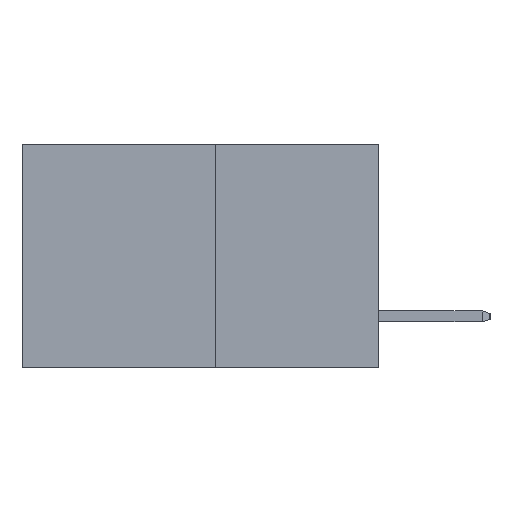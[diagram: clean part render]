
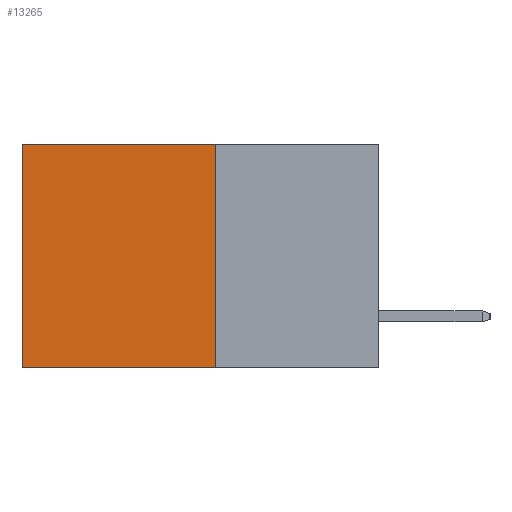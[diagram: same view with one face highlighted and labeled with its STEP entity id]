
A CAD part, left-side view. The second image highlights one B-rep face of the part: STEP entity #13265.
In plain terms, the highlighted planar face has unit normal (-1, 0, 0).
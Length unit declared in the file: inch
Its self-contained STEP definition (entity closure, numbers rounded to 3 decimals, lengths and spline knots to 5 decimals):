
#51 = EDGE_CURVE ( 'NONE', #7438, #7087, #12835, .T. ) ;
#212 = VECTOR ( 'NONE', #16253, 39.37008 ) ;
#741 = VERTEX_POINT ( 'NONE', #22607 ) ;
#2428 = LINE ( 'NONE', #10337, #6658 ) ;
#2478 = ORIENTED_EDGE ( 'NONE', *, *, #16968, .T. ) ;
#2841 = LINE ( 'NONE', #21409, #212 ) ;
#3084 = CARTESIAN_POINT ( 'NONE',  ( 0.277, 0.27, -0.37 ) ) ;
#3290 = DIRECTION ( 'NONE',  ( 0., 1., 0. ) ) ;
#3412 = VECTOR ( 'NONE', #17109, 39.37008 ) ;
#4464 = ORIENTED_EDGE ( 'NONE', *, *, #51, .F. ) ;
#5955 = FACE_OUTER_BOUND ( 'NONE', #7089, .T. ) ;
#6658 = VECTOR ( 'NONE', #3290, 39.37008 ) ;
#6681 = PLANE ( 'NONE',  #18501 ) ;
#7087 = VERTEX_POINT ( 'NONE', #18745 ) ;
#7089 = EDGE_LOOP ( 'NONE', ( #17391, #20608, #4464, #2478 ) ) ;
#7438 = VERTEX_POINT ( 'NONE', #10948 ) ;
#8458 = DIRECTION ( 'NONE',  ( 1., 0., 0. ) ) ;
#9931 = CARTESIAN_POINT ( 'NONE',  ( 0.277, 0.27, -0.37 ) ) ;
#10337 = CARTESIAN_POINT ( 'NONE',  ( 0.277, 0.27, -0.37 ) ) ;
#10948 = CARTESIAN_POINT ( 'NONE',  ( 0.277, 0.27, 0. ) ) ;
#11316 = LINE ( 'NONE', #16974, #20010 ) ;
#12835 = LINE ( 'NONE', #9931, #3412 ) ;
#13265 = ADVANCED_FACE ( 'NONE', ( #5955 ), #6681, .F. ) ;
#16253 = DIRECTION ( 'NONE',  ( 0., 0., -1. ) ) ;
#16856 = CARTESIAN_POINT ( 'NONE',  ( 0.277, 0.59, -0.37 ) ) ;
#16968 = EDGE_CURVE ( 'NONE', #7438, #741, #11316, .T. ) ;
#16974 = CARTESIAN_POINT ( 'NONE',  ( 0.277, 0.27, 0. ) ) ;
#17109 = DIRECTION ( 'NONE',  ( 0., 0., -1. ) ) ;
#17391 = ORIENTED_EDGE ( 'NONE', *, *, #20177, .T. ) ;
#18367 = VERTEX_POINT ( 'NONE', #16856 ) ;
#18501 = AXIS2_PLACEMENT_3D ( 'NONE', #3084, #8458, #20617 ) ;
#18698 = DIRECTION ( 'NONE',  ( 0., 1., 0. ) ) ;
#18745 = CARTESIAN_POINT ( 'NONE',  ( 0.277, 0.27, -0.37 ) ) ;
#20010 = VECTOR ( 'NONE', #18698, 39.37008 ) ;
#20177 = EDGE_CURVE ( 'NONE', #741, #18367, #2841, .T. ) ;
#20546 = EDGE_CURVE ( 'NONE', #7087, #18367, #2428, .T. ) ;
#20608 = ORIENTED_EDGE ( 'NONE', *, *, #20546, .F. ) ;
#20617 = DIRECTION ( 'NONE',  ( 0., 0., -1. ) ) ;
#21409 = CARTESIAN_POINT ( 'NONE',  ( 0.277, 0.59, -0.37 ) ) ;
#22607 = CARTESIAN_POINT ( 'NONE',  ( 0.277, 0.59, 0. ) ) ;
